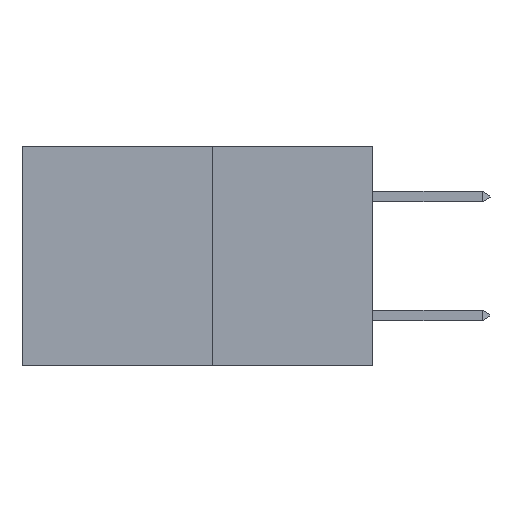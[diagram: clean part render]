
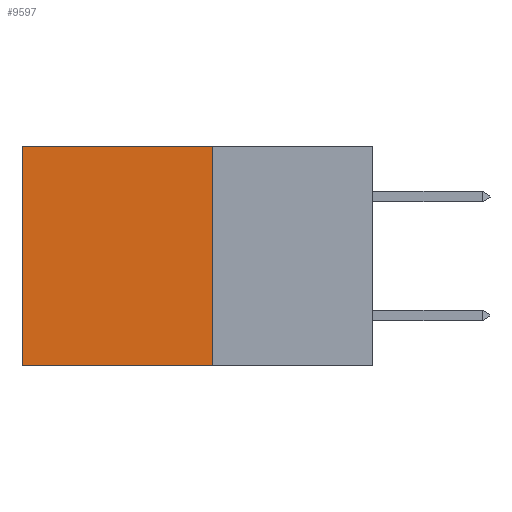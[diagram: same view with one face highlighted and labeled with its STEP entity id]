
A CAD part, left-side view. The second image highlights one B-rep face of the part: STEP entity #9597.
In plain terms, the highlighted planar face has unit normal (-1, 0, 0).
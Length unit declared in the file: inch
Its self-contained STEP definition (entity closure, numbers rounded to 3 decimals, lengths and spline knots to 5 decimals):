
#1226 = DIRECTION ( 'NONE',  ( 0., 0., -1. ) ) ;
#1228 = DIRECTION ( 'NONE',  ( 1., 0., 0. ) ) ;
#1243 = PLANE ( 'NONE',  #13243 ) ;
#1384 = CARTESIAN_POINT ( 'NONE',  ( 0.277, 0.27, -0.37 ) ) ;
#1818 = LINE ( 'NONE', #15550, #8414 ) ;
#1843 = VECTOR ( 'NONE', #6399, 39.37008 ) ;
#2098 = ORIENTED_EDGE ( 'NONE', *, *, #12420, .T. ) ;
#2226 = CARTESIAN_POINT ( 'NONE',  ( 0.277, 0.27, -0.37 ) ) ;
#2491 = EDGE_CURVE ( 'NONE', #8001, #15882, #12290, .T. ) ;
#4078 = CARTESIAN_POINT ( 'NONE',  ( 0.277, 0.59, -0.37 ) ) ;
#4653 = EDGE_CURVE ( 'NONE', #8001, #12704, #1818, .T. ) ;
#5038 = LINE ( 'NONE', #2226, #8566 ) ;
#5752 = CARTESIAN_POINT ( 'NONE',  ( 0.277, 0.27, -0.37 ) ) ;
#6062 = CARTESIAN_POINT ( 'NONE',  ( 0.277, 0.27, -0.37 ) ) ;
#6225 = ORIENTED_EDGE ( 'NONE', *, *, #12171, .F. ) ;
#6399 = DIRECTION ( 'NONE',  ( 0., 0., -1. ) ) ;
#7932 = VECTOR ( 'NONE', #13212, 39.37008 ) ;
#8001 = VERTEX_POINT ( 'NONE', #12284 ) ;
#8414 = VECTOR ( 'NONE', #15290, 39.37008 ) ;
#8566 = VECTOR ( 'NONE', #10042, 39.37008 ) ;
#9597 = ADVANCED_FACE ( 'NONE', ( #9892 ), #1243, .F. ) ;
#9860 = CARTESIAN_POINT ( 'NONE',  ( 0.277, 0.59, 0. ) ) ;
#9892 = FACE_OUTER_BOUND ( 'NONE', #11286, .T. ) ;
#10042 = DIRECTION ( 'NONE',  ( 0., 1., 0. ) ) ;
#10646 = ORIENTED_EDGE ( 'NONE', *, *, #2491, .F. ) ;
#11190 = ORIENTED_EDGE ( 'NONE', *, *, #4653, .T. ) ;
#11286 = EDGE_LOOP ( 'NONE', ( #2098, #6225, #10646, #11190 ) ) ;
#12171 = EDGE_CURVE ( 'NONE', #15882, #16475, #5038, .T. ) ;
#12284 = CARTESIAN_POINT ( 'NONE',  ( 0.277, 0.27, 0. ) ) ;
#12290 = LINE ( 'NONE', #6062, #1843 ) ;
#12420 = EDGE_CURVE ( 'NONE', #12704, #16475, #14443, .T. ) ;
#12704 = VERTEX_POINT ( 'NONE', #9860 ) ;
#13212 = DIRECTION ( 'NONE',  ( 0., 0., -1. ) ) ;
#13243 = AXIS2_PLACEMENT_3D ( 'NONE', #1384, #1228, #1226 ) ;
#14443 = LINE ( 'NONE', #4078, #7932 ) ;
#15290 = DIRECTION ( 'NONE',  ( 0., 1., 0. ) ) ;
#15550 = CARTESIAN_POINT ( 'NONE',  ( 0.277, 0.27, 0. ) ) ;
#15882 = VERTEX_POINT ( 'NONE', #5752 ) ;
#16393 = CARTESIAN_POINT ( 'NONE',  ( 0.277, 0.59, -0.37 ) ) ;
#16475 = VERTEX_POINT ( 'NONE', #16393 ) ;
